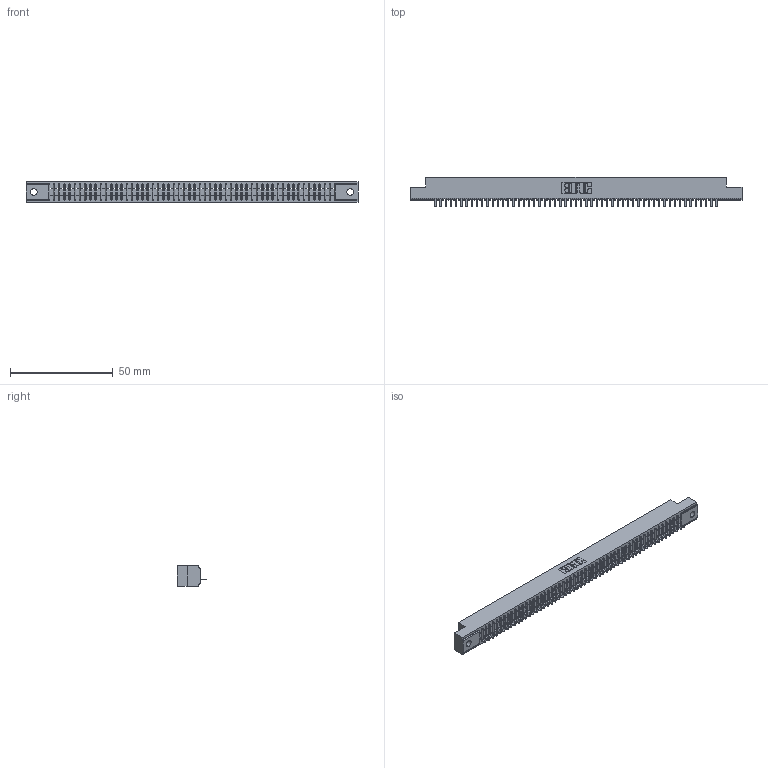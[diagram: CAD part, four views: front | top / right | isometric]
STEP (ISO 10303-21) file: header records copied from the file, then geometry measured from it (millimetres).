
FILE_DESCRIPTION (( 'STEP AP203' ), '1' );
FILE_NAME ('391-055-520-102.STEP', '2018-08-09T07:30:04', ( '' ), ( '' ), 'SwSTEP 2.0', 'SolidWorks 2016', '' );
FILE_SCHEMA (( 'CONFIG_CONTROL_DESIGN' ));
Length unit declared in the file: inch
Products named in the file (3): 341 Part_.128 (3.25) Dia Mounting Holes; 341-292-001_341-292-120; 391-055-520-102
Assembly tree (56 placements, depth 2):
  391-055-520-102
    341 Part_.128 (3.25) Dia Mounting Holes
    341-292-001_341-292-120  x55
Bounding box: 161.93 x 14.27 x 10.16 mm (x, y, z)
Volume: 11537.2 mm3; surface area: 17849.3 mm2
Topology: 56 solids, 56 shells, 4626 faces, 13351 edges, 8566 vertices
Faces by surface type: plane 2873, cylinder 1533, sphere 112, torus 108
Entity records: 63072 total; most frequent: CARTESIAN_POINT 10722, ORIENTED_EDGE 10710, DIRECTION 10339, EDGE_CURVE 5355, LINE 4341, VECTOR 4341, VERTEX_POINT 3382, AXIS2_PLACEMENT_3D 2999
